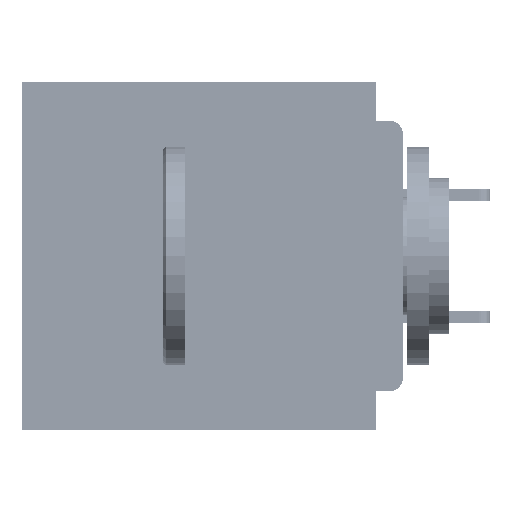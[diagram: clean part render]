
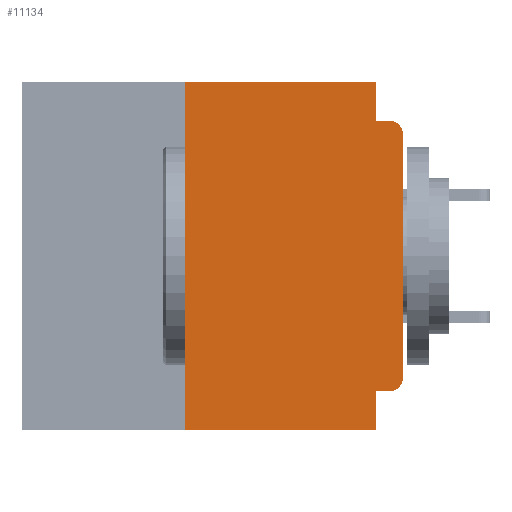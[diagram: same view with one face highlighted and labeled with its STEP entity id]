
A CAD part, left-side view. The second image highlights one B-rep face of the part: STEP entity #11134.
In plain terms, the highlighted planar face has unit normal (-1, 0, 0).
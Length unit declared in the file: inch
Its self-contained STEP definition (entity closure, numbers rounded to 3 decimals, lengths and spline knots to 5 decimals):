
#345 = LINE ( 'NONE', #69023, #42096 ) ;
#1243 = CARTESIAN_POINT ( 'NONE',  ( 0., 0.015, -0.045 ) ) ;
#1848 = CARTESIAN_POINT ( 'NONE',  ( 0., 0.25, 0. ) ) ;
#2346 = LINE ( 'NONE', #26021, #60122 ) ;
#2445 = CARTESIAN_POINT ( 'NONE',  ( 0., 0.031, 0. ) ) ;
#2883 = DIRECTION ( 'NONE',  ( -1., 0., 0. ) ) ;
#3447 = DIRECTION ( 'NONE',  ( 0., -1., 0. ) ) ;
#4401 = ORIENTED_EDGE ( 'NONE', *, *, #34418, .F. ) ;
#4961 = LINE ( 'NONE', #51923, #59314 ) ;
#5222 = FACE_OUTER_BOUND ( 'NONE', #15283, .T. ) ;
#5993 = DIRECTION ( 'NONE',  ( -1., 0., 0. ) ) ;
#6796 = VERTEX_POINT ( 'NONE', #58226 ) ;
#6858 = CIRCLE ( 'NONE', #39615, 0.015 ) ;
#7567 = VERTEX_POINT ( 'NONE', #21736 ) ;
#9524 = ORIENTED_EDGE ( 'NONE', *, *, #17046, .F. ) ;
#10932 = DIRECTION ( 'NONE',  ( 0., 0., -1. ) ) ;
#11134 = ADVANCED_FACE ( 'NONE', ( #5222 ), #37991, .F. ) ;
#12676 = VECTOR ( 'NONE', #3447, 39.37008 ) ;
#14464 = CARTESIAN_POINT ( 'NONE',  ( 0., 0., -0.045 ) ) ;
#15220 = CARTESIAN_POINT ( 'NONE',  ( 0., 0.031, 0. ) ) ;
#15283 = EDGE_LOOP ( 'NONE', ( #38280, #40695, #40293, #9524, #4401, #26857, #33096, #37486, #43061, #48523 ) ) ;
#17046 = EDGE_CURVE ( 'NONE', #52630, #42639, #18289, .T. ) ;
#18010 = EDGE_CURVE ( 'NONE', #7567, #21712, #36944, .T. ) ;
#18289 = LINE ( 'NONE', #15220, #29326 ) ;
#21712 = VERTEX_POINT ( 'NONE', #1243 ) ;
#21736 = CARTESIAN_POINT ( 'NONE',  ( 0., 0., -0.06 ) ) ;
#21931 = DIRECTION ( 'NONE',  ( 0., -1., 0. ) ) ;
#22625 = CARTESIAN_POINT ( 'NONE',  ( 0., 0., 0. ) ) ;
#22684 = CARTESIAN_POINT ( 'NONE',  ( 0., 0.25, -0.4 ) ) ;
#23894 = EDGE_CURVE ( 'NONE', #56819, #46396, #2346, .T. ) ;
#24152 = EDGE_CURVE ( 'NONE', #60055, #7567, #55887, .T. ) ;
#24345 = VERTEX_POINT ( 'NONE', #62838 ) ;
#25543 = LINE ( 'NONE', #22684, #60598 ) ;
#25721 = EDGE_CURVE ( 'NONE', #24345, #6796, #345, .T. ) ;
#26021 = CARTESIAN_POINT ( 'NONE',  ( 0., 0., -0.355 ) ) ;
#26857 = ORIENTED_EDGE ( 'NONE', *, *, #54259, .F. ) ;
#28200 = EDGE_CURVE ( 'NONE', #56819, #60055, #6858, .T. ) ;
#28824 = LINE ( 'NONE', #14464, #12676 ) ;
#29326 = VECTOR ( 'NONE', #47722, 39.37008 ) ;
#33096 = ORIENTED_EDGE ( 'NONE', *, *, #25721, .T. ) ;
#33256 = LINE ( 'NONE', #59843, #60373 ) ;
#34418 = EDGE_CURVE ( 'NONE', #44542, #52630, #33256, .T. ) ;
#35496 = CARTESIAN_POINT ( 'NONE',  ( 0., 0.015, -0.06 ) ) ;
#36944 = CIRCLE ( 'NONE', #56763, 0.015 ) ;
#37486 = ORIENTED_EDGE ( 'NONE', *, *, #55611, .F. ) ;
#37991 = PLANE ( 'NONE',  #67181 ) ;
#38280 = ORIENTED_EDGE ( 'NONE', *, *, #24152, .T. ) ;
#38565 = CARTESIAN_POINT ( 'NONE',  ( 0., 0.015, -0.34 ) ) ;
#38734 = CARTESIAN_POINT ( 'NONE',  ( 0., 0.031, -0.045 ) ) ;
#39615 = AXIS2_PLACEMENT_3D ( 'NONE', #38565, #5993, #44036 ) ;
#40293 = ORIENTED_EDGE ( 'NONE', *, *, #55691, .F. ) ;
#40695 = ORIENTED_EDGE ( 'NONE', *, *, #18010, .T. ) ;
#40925 = DIRECTION ( 'NONE',  ( 0., 0., -1. ) ) ;
#41464 = VECTOR ( 'NONE', #55113, 39.37008 ) ;
#42096 = VECTOR ( 'NONE', #47446, 39.37008 ) ;
#42639 = VERTEX_POINT ( 'NONE', #38734 ) ;
#43061 = ORIENTED_EDGE ( 'NONE', *, *, #23894, .F. ) ;
#43444 = DIRECTION ( 'NONE',  ( 1., 0., 0. ) ) ;
#44036 = DIRECTION ( 'NONE',  ( 0., 0., -1. ) ) ;
#44531 = DIRECTION ( 'NONE',  ( 0., 0., 1. ) ) ;
#44542 = VERTEX_POINT ( 'NONE', #1848 ) ;
#46396 = VERTEX_POINT ( 'NONE', #59278 ) ;
#47446 = DIRECTION ( 'NONE',  ( 0., -1., 0. ) ) ;
#47722 = DIRECTION ( 'NONE',  ( 0., 0., -1. ) ) ;
#48451 = CARTESIAN_POINT ( 'NONE',  ( 0., 0., -0.34 ) ) ;
#48523 = ORIENTED_EDGE ( 'NONE', *, *, #28200, .T. ) ;
#51923 = CARTESIAN_POINT ( 'NONE',  ( 0., 0.031, -0.4 ) ) ;
#52630 = VERTEX_POINT ( 'NONE', #2445 ) ;
#54259 = EDGE_CURVE ( 'NONE', #24345, #44542, #25543, .T. ) ;
#54359 = CARTESIAN_POINT ( 'NONE',  ( 0., 0.015, -0.355 ) ) ;
#55113 = DIRECTION ( 'NONE',  ( 0., 0., 1. ) ) ;
#55611 = EDGE_CURVE ( 'NONE', #46396, #6796, #4961, .T. ) ;
#55691 = EDGE_CURVE ( 'NONE', #42639, #21712, #28824, .T. ) ;
#55887 = LINE ( 'NONE', #22625, #41464 ) ;
#56763 = AXIS2_PLACEMENT_3D ( 'NONE', #35496, #2883, #40925 ) ;
#56819 = VERTEX_POINT ( 'NONE', #54359 ) ;
#57386 = DIRECTION ( 'NONE',  ( 0., 0., -1. ) ) ;
#58226 = CARTESIAN_POINT ( 'NONE',  ( 0., 0.031, -0.4 ) ) ;
#58465 = DIRECTION ( 'NONE',  ( 0., 1., 0. ) ) ;
#59278 = CARTESIAN_POINT ( 'NONE',  ( 0., 0.031, -0.355 ) ) ;
#59314 = VECTOR ( 'NONE', #57386, 39.37008 ) ;
#59843 = CARTESIAN_POINT ( 'NONE',  ( 0., 0.437, 0. ) ) ;
#60055 = VERTEX_POINT ( 'NONE', #48451 ) ;
#60122 = VECTOR ( 'NONE', #58465, 39.37008 ) ;
#60373 = VECTOR ( 'NONE', #21931, 39.37008 ) ;
#60598 = VECTOR ( 'NONE', #44531, 39.37008 ) ;
#62838 = CARTESIAN_POINT ( 'NONE',  ( 0., 0.25, -0.4 ) ) ;
#67181 = AXIS2_PLACEMENT_3D ( 'NONE', #69630, #43444, #10932 ) ;
#69023 = CARTESIAN_POINT ( 'NONE',  ( 0., 0.437, -0.4 ) ) ;
#69630 = CARTESIAN_POINT ( 'NONE',  ( 0., 0.437, 0. ) ) ;
